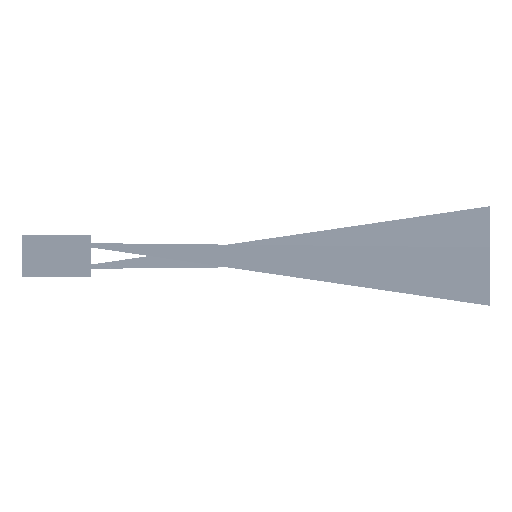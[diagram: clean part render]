
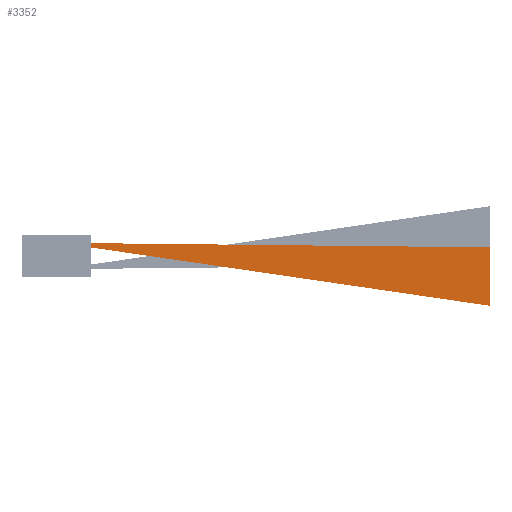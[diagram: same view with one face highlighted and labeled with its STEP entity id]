
A CAD part, left-side view. The second image highlights one B-rep face of the part: STEP entity #3352.
In plain terms, the highlighted face is planar.
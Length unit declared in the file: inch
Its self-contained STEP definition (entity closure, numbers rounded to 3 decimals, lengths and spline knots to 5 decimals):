
#389 = LINE ( 'NONE', #33869, #31860 ) ;
#414 = ORIENTED_EDGE ( 'NONE', *, *, #43932, .T. ) ;
#667 = DIRECTION ( 'NONE',  ( 1., 0., 0. ) ) ;
#924 = LINE ( 'NONE', #18521, #6067 ) ;
#1364 = ORIENTED_EDGE ( 'NONE', *, *, #40296, .F. ) ;
#1514 = FACE_OUTER_BOUND ( 'NONE', #50752, .T. ) ;
#2080 = CARTESIAN_POINT ( 'NONE',  ( 0.33619, 0.044, -0.025 ) ) ;
#2751 = DIRECTION ( 'NONE',  ( 0., 0., 1. ) ) ;
#3054 = CARTESIAN_POINT ( 'NONE',  ( 0.14781, 0.08118, -0.025 ) ) ;
#3352 = ADVANCED_FACE ( 'NONE', ( #1514 ), #43683, .F. ) ;
#3661 = DIRECTION ( 'NONE',  ( 1., 0., 0. ) ) ;
#3872 = VERTEX_POINT ( 'NONE', #26404 ) ;
#4990 = EDGE_CURVE ( 'NONE', #47604, #3872, #45683, .T. ) ;
#5165 = VERTEX_POINT ( 'NONE', #17683 ) ;
#6067 = VECTOR ( 'NONE', #26201, 39.37008 ) ;
#6288 = EDGE_CURVE ( 'NONE', #36062, #46447, #25848, .T. ) ;
#6348 = VECTOR ( 'NONE', #27534, 39.37008 ) ;
#6642 = DIRECTION ( 'NONE',  ( 1., 0., 0. ) ) ;
#7056 = AXIS2_PLACEMENT_3D ( 'NONE', #44681, #31907, #32261 ) ;
#7664 = LINE ( 'NONE', #31221, #17320 ) ;
#7898 = DIRECTION ( 'NONE',  ( 0.893, 0.449, 0. ) ) ;
#8396 = DIRECTION ( 'NONE',  ( 1., 0., 0. ) ) ;
#8694 = AXIS2_PLACEMENT_3D ( 'NONE', #2080, #22420, #38312 ) ;
#8741 = DIRECTION ( 'NONE',  ( -1., 0., 0. ) ) ;
#9084 = CARTESIAN_POINT ( 'NONE',  ( 0.13321, 0.058, -0.025 ) ) ;
#9967 = EDGE_CURVE ( 'NONE', #21212, #10486, #17111, .T. ) ;
#10006 = ORIENTED_EDGE ( 'NONE', *, *, #9967, .T. ) ;
#10248 = ORIENTED_EDGE ( 'NONE', *, *, #25281, .F. ) ;
#10486 = VERTEX_POINT ( 'NONE', #38756 ) ;
#10934 = VERTEX_POINT ( 'NONE', #25220 ) ;
#11790 = DIRECTION ( 'NONE',  ( 0., -1., 0. ) ) ;
#12056 = CARTESIAN_POINT ( 'NONE',  ( 0.43721, 0.04723, -0.025 ) ) ;
#12969 = CIRCLE ( 'NONE', #22863, 0.0635 ) ;
#14892 = CARTESIAN_POINT ( 'NONE',  ( 0.30469, 0.0435, -0.025 ) ) ;
#16958 = CARTESIAN_POINT ( 'NONE',  ( 0.43721, 0.0255, -0.025 ) ) ;
#16962 = EDGE_CURVE ( 'NONE', #18537, #17113, #12969, .T. ) ;
#17111 = CIRCLE ( 'NONE', #49927, 0.0185 ) ;
#17113 = VERTEX_POINT ( 'NONE', #14892 ) ;
#17320 = VECTOR ( 'NONE', #6642, 39.37008 ) ;
#17683 = CARTESIAN_POINT ( 'NONE',  ( 0.58021, 0.0375, -0.025 ) ) ;
#18521 = CARTESIAN_POINT ( 'NONE',  ( 0.15365, 0.06956, -0.025 ) ) ;
#18537 = VERTEX_POINT ( 'NONE', #44545 ) ;
#18783 = VERTEX_POINT ( 'NONE', #50281 ) ;
#19489 = DIRECTION ( 'NONE',  ( 0., 0., 1. ) ) ;
#20060 = VERTEX_POINT ( 'NONE', #41364 ) ;
#20062 = CARTESIAN_POINT ( 'NONE',  ( 0.45258, 0.03186, -0.025 ) ) ;
#20113 = AXIS2_PLACEMENT_3D ( 'NONE', #35908, #2751, #43334 ) ;
#20157 = DIRECTION ( 'NONE',  ( 0., 0., 1. ) ) ;
#20402 = AXIS2_PLACEMENT_3D ( 'NONE', #20992, #49688, #8741 ) ;
#20825 = CIRCLE ( 'NONE', #7056, 0.0765 ) ;
#20923 = ORIENTED_EDGE ( 'NONE', *, *, #16962, .F. ) ;
#20975 = EDGE_CURVE ( 'NONE', #10486, #24909, #7664, .T. ) ;
#20992 = CARTESIAN_POINT ( 'NONE',  ( 0.15971, 0.0575, -0.025 ) ) ;
#20993 = ORIENTED_EDGE ( 'NONE', *, *, #33136, .T. ) ;
#21212 = VERTEX_POINT ( 'NONE', #28835 ) ;
#21291 = VECTOR ( 'NONE', #29138, 39.37008 ) ;
#21625 = ORIENTED_EDGE ( 'NONE', *, *, #41346, .F. ) ;
#21804 = VERTEX_POINT ( 'NONE', #20062 ) ;
#21872 = CARTESIAN_POINT ( 'NONE',  ( 4.1375, 0.558, -0.0725 ) ) ;
#22420 = DIRECTION ( 'NONE',  ( 0., 0., 1. ) ) ;
#22863 = AXIS2_PLACEMENT_3D ( 'NONE', #38375, #26544, #26731 ) ;
#23457 = CARTESIAN_POINT ( 'NONE',  ( 0.58021, 0.016, -0.025 ) ) ;
#23621 = CARTESIAN_POINT ( 'NONE',  ( 0.33619, 0.044, -0.025 ) ) ;
#24274 = VERTEX_POINT ( 'NONE', #33153 ) ;
#24909 = VERTEX_POINT ( 'NONE', #16958 ) ;
#25220 = CARTESIAN_POINT ( 'NONE',  ( 0.33619, 0.0125, -0.025 ) ) ;
#25281 = EDGE_CURVE ( 'NONE', #47604, #44234, #39580, .T. ) ;
#25362 = ORIENTED_EDGE ( 'NONE', *, *, #20975, .T. ) ;
#25378 = ORIENTED_EDGE ( 'NONE', *, *, #31128, .T. ) ;
#25848 = LINE ( 'NONE', #27734, #41913 ) ;
#26201 = DIRECTION ( 'NONE',  ( 0.893, 0.449, 0. ) ) ;
#26404 = CARTESIAN_POINT ( 'NONE',  ( 0.13322, 0.058, -0.025 ) ) ;
#26544 = DIRECTION ( 'NONE',  ( 0., 0., -1. ) ) ;
#26572 = LINE ( 'NONE', #3054, #47831 ) ;
#26731 = DIRECTION ( 'NONE',  ( -1., 0., 0. ) ) ;
#26980 = DIRECTION ( 'NONE',  ( -1., 0., 0. ) ) ;
#27159 = ORIENTED_EDGE ( 'NONE', *, *, #48123, .F. ) ;
#27316 = CARTESIAN_POINT ( 'NONE',  ( 0.15971, 0.0575, -0.025 ) ) ;
#27491 = DIRECTION ( 'NONE',  ( 0., 0., -1. ) ) ;
#27534 = DIRECTION ( 'NONE',  ( 0., 1., 0. ) ) ;
#27535 = LINE ( 'NONE', #23457, #6348 ) ;
#27734 = CARTESIAN_POINT ( 'NONE',  ( 4.1375, 0.6, -0.0725 ) ) ;
#28835 = CARTESIAN_POINT ( 'NONE',  ( 0.31769, 0.04371, -0.025 ) ) ;
#28905 = CARTESIAN_POINT ( 'NONE',  ( 4.1375, 0.05, -0.0725 ) ) ;
#29138 = DIRECTION ( 'NONE',  ( -1., 0., 0. ) ) ;
#30673 = CARTESIAN_POINT ( 'NONE',  ( 0.14622, 0.058, -0.025 ) ) ;
#31128 = EDGE_CURVE ( 'NONE', #24909, #21804, #32089, .T. ) ;
#31221 = CARTESIAN_POINT ( 'NONE',  ( 0.33619, 0.0255, -0.025 ) ) ;
#31860 = VECTOR ( 'NONE', #667, 39.37008 ) ;
#31907 = DIRECTION ( 'NONE',  ( 0., 0., -1. ) ) ;
#32089 = CIRCLE ( 'NONE', #46013, 0.02173 ) ;
#32261 = DIRECTION ( 'NONE',  ( -1., 0., 0. ) ) ;
#32972 = CARTESIAN_POINT ( 'NONE',  ( 0.33619, 0.0125, -0.025 ) ) ;
#33136 = EDGE_CURVE ( 'NONE', #38526, #5165, #389, .T. ) ;
#33153 = CARTESIAN_POINT ( 'NONE',  ( 0.14781, 0.08118, -0.025 ) ) ;
#33869 = CARTESIAN_POINT ( 'NONE',  ( 0.45821, 0.0375, -0.025 ) ) ;
#35198 = EDGE_CURVE ( 'NONE', #24274, #20060, #26572, .T. ) ;
#35908 = CARTESIAN_POINT ( 'NONE',  ( 0.095, 0.025, -0.025 ) ) ;
#36062 = VERTEX_POINT ( 'NONE', #21872 ) ;
#37479 = AXIS2_PLACEMENT_3D ( 'NONE', #27316, #27491, #26980 ) ;
#38019 = EDGE_CURVE ( 'NONE', #18783, #5165, #27535, .T. ) ;
#38312 = DIRECTION ( 'NONE',  ( 1., 0., 0. ) ) ;
#38375 = CARTESIAN_POINT ( 'NONE',  ( 0.2412, 0.0425, -0.025 ) ) ;
#38526 = VERTEX_POINT ( 'NONE', #38538 ) ;
#38538 = CARTESIAN_POINT ( 'NONE',  ( 0.45821, 0.0375, -0.025 ) ) ;
#38756 = CARTESIAN_POINT ( 'NONE',  ( 0.33619, 0.0255, -0.025 ) ) ;
#38865 = CARTESIAN_POINT ( 'NONE',  ( 0.15365, 0.06956, -0.025 ) ) ;
#39580 = CIRCLE ( 'NONE', #37479, 0.0135 ) ;
#40296 = EDGE_CURVE ( 'NONE', #44234, #18537, #924, .T. ) ;
#40699 = ORIENTED_EDGE ( 'NONE', *, *, #50891, .T. ) ;
#41346 = EDGE_CURVE ( 'NONE', #17113, #10934, #44582, .T. ) ;
#41354 = ORIENTED_EDGE ( 'NONE', *, *, #6288, .F. ) ;
#41364 = CARTESIAN_POINT ( 'NONE',  ( 0.20684, 0.11085, -0.025 ) ) ;
#41532 = ORIENTED_EDGE ( 'NONE', *, *, #4990, .T. ) ;
#41881 = CIRCLE ( 'NONE', #20402, 0.0265 ) ;
#41913 = VECTOR ( 'NONE', #11790, 39.37008 ) ;
#43334 = DIRECTION ( 'NONE',  ( 1., 0., 0. ) ) ;
#43683 = PLANE ( 'NONE',  #20113 ) ;
#43686 = ORIENTED_EDGE ( 'NONE', *, *, #35198, .T. ) ;
#43932 = EDGE_CURVE ( 'NONE', #20060, #21212, #20825, .T. ) ;
#44234 = VERTEX_POINT ( 'NONE', #38865 ) ;
#44545 = CARTESIAN_POINT ( 'NONE',  ( 0.21268, 0.09924, -0.025 ) ) ;
#44582 = CIRCLE ( 'NONE', #8694, 0.0315 ) ;
#44681 = CARTESIAN_POINT ( 'NONE',  ( 0.2412, 0.0425, -0.025 ) ) ;
#44899 = DIRECTION ( 'NONE',  ( 1., 0., 0. ) ) ;
#45683 = LINE ( 'NONE', #9084, #21291 ) ;
#45688 = ORIENTED_EDGE ( 'NONE', *, *, #38019, .F. ) ;
#46013 = AXIS2_PLACEMENT_3D ( 'NONE', #12056, #20157, #44899 ) ;
#46227 = LINE ( 'NONE', #32972, #51399 ) ;
#46447 = VERTEX_POINT ( 'NONE', #28905 ) ;
#47593 = ORIENTED_EDGE ( 'NONE', *, *, #41354, .T. ) ;
#47604 = VERTEX_POINT ( 'NONE', #30673 ) ;
#47831 = VECTOR ( 'NONE', #7898, 39.37008 ) ;
#48123 = EDGE_CURVE ( 'NONE', #10934, #18783, #46227, .T. ) ;
#49688 = DIRECTION ( 'NONE',  ( 0., 0., -1. ) ) ;
#49927 = AXIS2_PLACEMENT_3D ( 'NONE', #23621, #19489, #3661 ) ;
#50281 = CARTESIAN_POINT ( 'NONE',  ( 0.58021, 0.0125, -0.025 ) ) ;
#50752 = EDGE_LOOP ( 'NONE', ( #10248, #41532, #40699, #43686, #414, #10006, #25362, #25378, #47593, #20993, #45688, #27159, #21625, #20923, #1364 ) ) ;
#50891 = EDGE_CURVE ( 'NONE', #3872, #24274, #41881, .T. ) ;
#51399 = VECTOR ( 'NONE', #8396, 39.37008 ) ;
